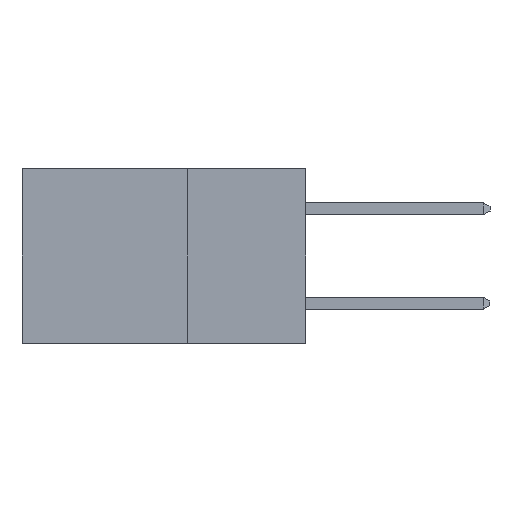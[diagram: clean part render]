
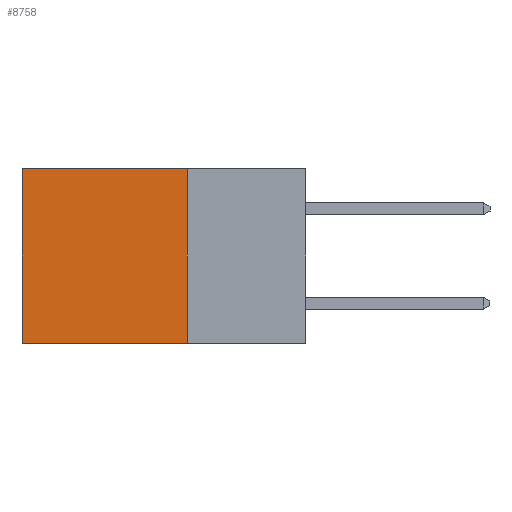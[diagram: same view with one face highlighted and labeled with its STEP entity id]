
A CAD part, left-side view. The second image highlights one B-rep face of the part: STEP entity #8758.
In plain terms, the highlighted planar face has unit normal (-1, 0, 0).
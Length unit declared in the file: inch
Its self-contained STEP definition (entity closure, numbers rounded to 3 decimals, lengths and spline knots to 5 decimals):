
#55 = VECTOR ( 'NONE', #15263, 39.37008 ) ;
#64 = LINE ( 'NONE', #17120, #14292 ) ;
#1653 = CARTESIAN_POINT ( 'NONE',  ( 0.298, 0.25, 0. ) ) ;
#1945 = EDGE_LOOP ( 'NONE', ( #7938, #7780, #17428, #16262 ) ) ;
#2447 = EDGE_CURVE ( 'NONE', #5607, #14042, #14415, .T. ) ;
#2560 = EDGE_CURVE ( 'NONE', #14042, #13889, #15853, .T. ) ;
#2566 = AXIS2_PLACEMENT_3D ( 'NONE', #13912, #15244, #7020 ) ;
#3369 = VECTOR ( 'NONE', #13475, 39.37008 ) ;
#3645 = CARTESIAN_POINT ( 'NONE',  ( 0.298, 0.6, 0. ) ) ;
#3937 = CARTESIAN_POINT ( 'NONE',  ( 0.298, 0.6, -0.37 ) ) ;
#4217 = PLANE ( 'NONE',  #2566 ) ;
#4719 = CARTESIAN_POINT ( 'NONE',  ( 0.298, 0.25, 0. ) ) ;
#4739 = CARTESIAN_POINT ( 'NONE',  ( 0.298, 0.25, -0.37 ) ) ;
#4893 = DIRECTION ( 'NONE',  ( 0., 1., 0. ) ) ;
#5607 = VERTEX_POINT ( 'NONE', #1653 ) ;
#5627 = CARTESIAN_POINT ( 'NONE',  ( 0.298, 0.25, 0. ) ) ;
#7020 = DIRECTION ( 'NONE',  ( 0., 0., -1. ) ) ;
#7637 = DIRECTION ( 'NONE',  ( 0., 0., -1. ) ) ;
#7780 = ORIENTED_EDGE ( 'NONE', *, *, #2560, .F. ) ;
#7938 = ORIENTED_EDGE ( 'NONE', *, *, #9089, .T. ) ;
#8758 = ADVANCED_FACE ( 'NONE', ( #12159 ), #4217, .F. ) ;
#9089 = EDGE_CURVE ( 'NONE', #10412, #13889, #64, .T. ) ;
#10412 = VERTEX_POINT ( 'NONE', #3645 ) ;
#12159 = FACE_OUTER_BOUND ( 'NONE', #1945, .T. ) ;
#12267 = VECTOR ( 'NONE', #4893, 39.37008 ) ;
#13475 = DIRECTION ( 'NONE',  ( 0., 0., -1. ) ) ;
#13889 = VERTEX_POINT ( 'NONE', #3937 ) ;
#13912 = CARTESIAN_POINT ( 'NONE',  ( 0.298, 0.25, 0. ) ) ;
#13943 = CARTESIAN_POINT ( 'NONE',  ( 0.298, 0.25, -0.37 ) ) ;
#14042 = VERTEX_POINT ( 'NONE', #13943 ) ;
#14287 = LINE ( 'NONE', #5627, #55 ) ;
#14292 = VECTOR ( 'NONE', #7637, 39.37008 ) ;
#14415 = LINE ( 'NONE', #4719, #3369 ) ;
#15244 = DIRECTION ( 'NONE',  ( 1., 0., 0. ) ) ;
#15263 = DIRECTION ( 'NONE',  ( 0., 1., 0. ) ) ;
#15853 = LINE ( 'NONE', #4739, #12267 ) ;
#15917 = EDGE_CURVE ( 'NONE', #5607, #10412, #14287, .T. ) ;
#16262 = ORIENTED_EDGE ( 'NONE', *, *, #15917, .T. ) ;
#17120 = CARTESIAN_POINT ( 'NONE',  ( 0.298, 0.6, 0. ) ) ;
#17428 = ORIENTED_EDGE ( 'NONE', *, *, #2447, .F. ) ;
